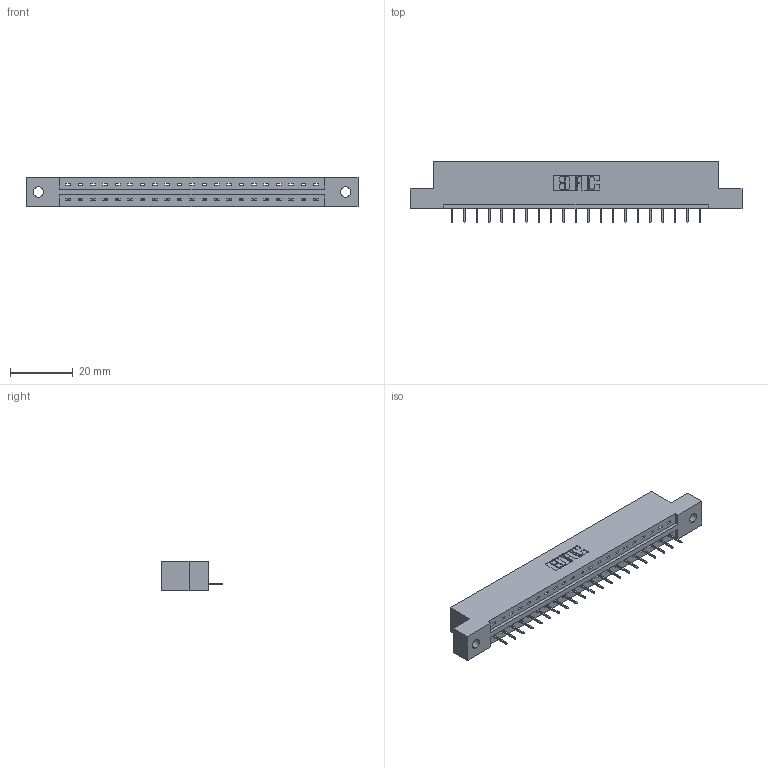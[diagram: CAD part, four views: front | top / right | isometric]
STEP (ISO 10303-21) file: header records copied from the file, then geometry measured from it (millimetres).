
FILE_DESCRIPTION (( 'STEP AP203' ), '1' );
FILE_NAME ('337-021-524-102.STEP', '2018-08-05T11:25:39', ( '' ), ( '' ), 'SwSTEP 2.0', 'SolidWorks 2016', '' );
FILE_SCHEMA (( 'CONFIG_CONTROL_DESIGN' ));
Length unit declared in the file: inch
Products named in the file (3): 337 Part_Flush Mounting Lugs - 0.128 Dia; 345-292-001_345-293-124; 337-021-524-102
Assembly tree (22 placements, depth 2):
  337-021-524-102
    337 Part_Flush Mounting Lugs - 0.128 Dia
    345-292-001_345-293-124  x21
Bounding box: 106.22 x 19.69 x 9.4 mm (x, y, z)
Volume: 10657.6 mm3; surface area: 10335 mm2
Topology: 22 solids, 22 shells, 1500 faces, 4343 edges, 2810 vertices
Faces by surface type: plane 1162, cylinder 338
Entity records: 18403 total; most frequent: CARTESIAN_POINT 3209, ORIENTED_EDGE 3166, DIRECTION 2745, EDGE_CURVE 1583, LINE 1459, VECTOR 1459, VERTEX_POINT 1050, AXIS2_PLACEMENT_3D 643
